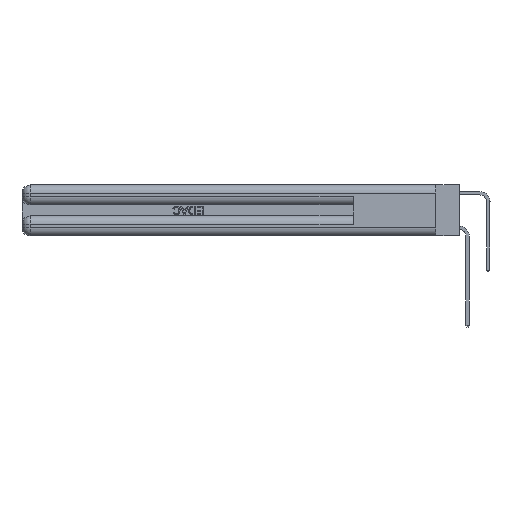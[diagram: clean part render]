
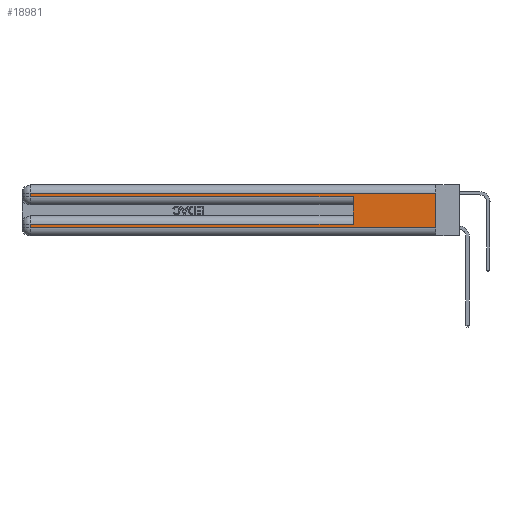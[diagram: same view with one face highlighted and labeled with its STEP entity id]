
A CAD part, left-side view. The second image highlights one B-rep face of the part: STEP entity #18981.
In plain terms, the highlighted planar face has unit normal (-1, 0, 0).
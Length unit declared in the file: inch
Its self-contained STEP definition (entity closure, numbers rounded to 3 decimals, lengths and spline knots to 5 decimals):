
#1387 = CARTESIAN_POINT ( 'NONE',  ( 0., 2.94, 0.31 ) ) ;
#1561 = DIRECTION ( 'NONE',  ( 0., 0., -1. ) ) ;
#2458 = ORIENTED_EDGE ( 'NONE', *, *, #15265, .T. ) ;
#2642 = CARTESIAN_POINT ( 'NONE',  ( 0., 0., 0.285 ) ) ;
#3376 = VECTOR ( 'NONE', #32348, 39.37008 ) ;
#3547 = CARTESIAN_POINT ( 'NONE',  ( 0., 0., 0.31 ) ) ;
#5512 = EDGE_CURVE ( 'NONE', #8745, #28424, #8474, .T. ) ;
#7494 = AXIS2_PLACEMENT_3D ( 'NONE', #15620, #18483, #1561 ) ;
#7804 = CARTESIAN_POINT ( 'NONE',  ( 0., 0.6, 0.085 ) ) ;
#8474 = LINE ( 'NONE', #2642, #12776 ) ;
#8745 = VERTEX_POINT ( 'NONE', #10000 ) ;
#10000 = CARTESIAN_POINT ( 'NONE',  ( 0., 2.94, 0.285 ) ) ;
#11311 = ORIENTED_EDGE ( 'NONE', *, *, #18292, .T. ) ;
#12776 = VECTOR ( 'NONE', #17080, 39.37008 ) ;
#13741 = ORIENTED_EDGE ( 'NONE', *, *, #16984, .T. ) ;
#14082 = VERTEX_POINT ( 'NONE', #34543 ) ;
#14898 = VECTOR ( 'NONE', #20922, 39.37008 ) ;
#15150 = ORIENTED_EDGE ( 'NONE', *, *, #25286, .F. ) ;
#15203 = CARTESIAN_POINT ( 'NONE',  ( 0., 0., 0.37 ) ) ;
#15265 = EDGE_CURVE ( 'NONE', #31323, #27579, #22242, .T. ) ;
#15455 = DIRECTION ( 'NONE',  ( 0., 0., -1. ) ) ;
#15620 = CARTESIAN_POINT ( 'NONE',  ( 0., 0., 0.37 ) ) ;
#16333 = ORIENTED_EDGE ( 'NONE', *, *, #30730, .F. ) ;
#16984 = EDGE_CURVE ( 'NONE', #27579, #8745, #25221, .T. ) ;
#17080 = DIRECTION ( 'NONE',  ( 0., -1., 0. ) ) ;
#18100 = CARTESIAN_POINT ( 'NONE',  ( 0., 0.6, 0.145 ) ) ;
#18292 = EDGE_CURVE ( 'NONE', #14082, #22715, #34435, .T. ) ;
#18483 = DIRECTION ( 'NONE',  ( 1., 0., 0. ) ) ;
#18981 = ADVANCED_FACE ( 'NONE', ( #28173 ), #32612, .F. ) ;
#19044 = CARTESIAN_POINT ( 'NONE',  ( 0., 0., 0.06 ) ) ;
#19407 = CARTESIAN_POINT ( 'NONE',  ( 0., 0., 0.31 ) ) ;
#20095 = DIRECTION ( 'NONE',  ( 0., 1., 0. ) ) ;
#20482 = ORIENTED_EDGE ( 'NONE', *, *, #21363, .T. ) ;
#20922 = DIRECTION ( 'NONE',  ( 0., -1., 0. ) ) ;
#20978 = LINE ( 'NONE', #24209, #29806 ) ;
#21029 = DIRECTION ( 'NONE',  ( 0., 0., -1. ) ) ;
#21363 = EDGE_CURVE ( 'NONE', #34917, #21391, #20978, .T. ) ;
#21391 = VERTEX_POINT ( 'NONE', #24926 ) ;
#21510 = ORIENTED_EDGE ( 'NONE', *, *, #36419, .T. ) ;
#22141 = VECTOR ( 'NONE', #21029, 39.37008 ) ;
#22242 = LINE ( 'NONE', #3547, #32866 ) ;
#22715 = VERTEX_POINT ( 'NONE', #19044 ) ;
#22841 = CARTESIAN_POINT ( 'NONE',  ( 0., 2.94, 0.37 ) ) ;
#23603 = LINE ( 'NONE', #15203, #24483 ) ;
#24209 = CARTESIAN_POINT ( 'NONE',  ( 0., 0., 0.085 ) ) ;
#24483 = VECTOR ( 'NONE', #15455, 39.37008 ) ;
#24926 = CARTESIAN_POINT ( 'NONE',  ( 0., 2.94, 0.085 ) ) ;
#25221 = LINE ( 'NONE', #32034, #22141 ) ;
#25286 = EDGE_CURVE ( 'NONE', #34917, #28424, #25958, .T. ) ;
#25958 = LINE ( 'NONE', #18100, #3376 ) ;
#26719 = CARTESIAN_POINT ( 'NONE',  ( 0., 0., 0.06 ) ) ;
#27229 = EDGE_LOOP ( 'NONE', ( #16333, #2458, #13741, #30601, #15150, #20482, #21510, #11311 ) ) ;
#27579 = VERTEX_POINT ( 'NONE', #1387 ) ;
#28173 = FACE_OUTER_BOUND ( 'NONE', #27229, .T. ) ;
#28424 = VERTEX_POINT ( 'NONE', #29871 ) ;
#29806 = VECTOR ( 'NONE', #30514, 39.37008 ) ;
#29871 = CARTESIAN_POINT ( 'NONE',  ( 0., 0.6, 0.285 ) ) ;
#30514 = DIRECTION ( 'NONE',  ( 0., 1., 0. ) ) ;
#30601 = ORIENTED_EDGE ( 'NONE', *, *, #5512, .T. ) ;
#30730 = EDGE_CURVE ( 'NONE', #31323, #22715, #23603, .T. ) ;
#30917 = DIRECTION ( 'NONE',  ( 0., 0., -1. ) ) ;
#31323 = VERTEX_POINT ( 'NONE', #19407 ) ;
#32034 = CARTESIAN_POINT ( 'NONE',  ( 0., 2.94, 0.37 ) ) ;
#32348 = DIRECTION ( 'NONE',  ( 0., 0., 1. ) ) ;
#32612 = PLANE ( 'NONE',  #7494 ) ;
#32784 = VECTOR ( 'NONE', #30917, 39.37008 ) ;
#32866 = VECTOR ( 'NONE', #20095, 39.37008 ) ;
#34435 = LINE ( 'NONE', #26719, #14898 ) ;
#34543 = CARTESIAN_POINT ( 'NONE',  ( 0., 2.94, 0.06 ) ) ;
#34578 = LINE ( 'NONE', #22841, #32784 ) ;
#34917 = VERTEX_POINT ( 'NONE', #7804 ) ;
#36419 = EDGE_CURVE ( 'NONE', #21391, #14082, #34578, .T. ) ;
